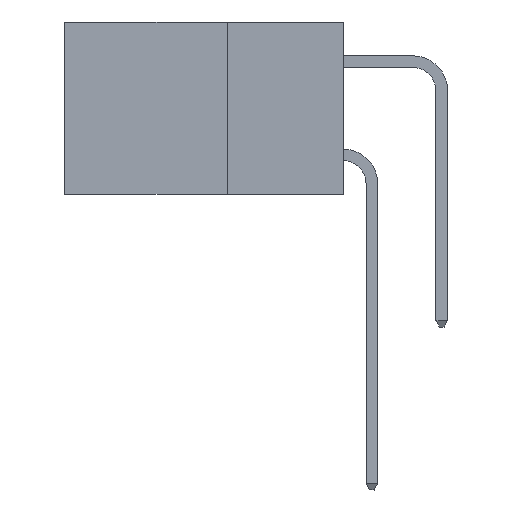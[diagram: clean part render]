
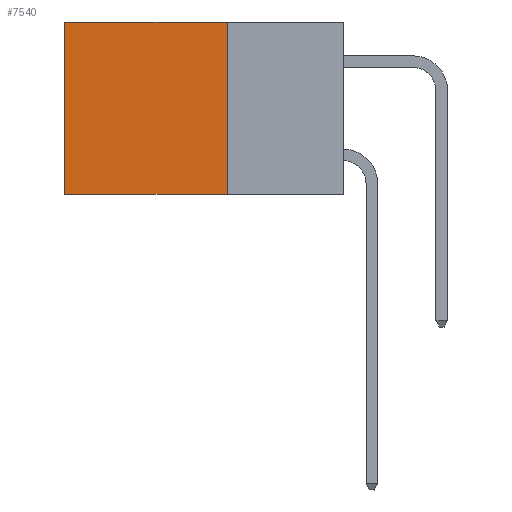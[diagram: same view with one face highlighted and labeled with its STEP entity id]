
A CAD part, left-side view. The second image highlights one B-rep face of the part: STEP entity #7540.
In plain terms, the highlighted planar face has unit normal (-1, 0, 0).
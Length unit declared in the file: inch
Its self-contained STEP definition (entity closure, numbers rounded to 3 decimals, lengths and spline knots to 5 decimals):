
#736 = AXIS2_PLACEMENT_3D ( 'NONE', #2807, #9020, #8856 ) ;
#985 = EDGE_LOOP ( 'NONE', ( #10716, #6815, #7611, #10050 ) ) ;
#1026 = CARTESIAN_POINT ( 'NONE',  ( 0.2615, 0.6, -0.37 ) ) ;
#2457 = VECTOR ( 'NONE', #3982, 39.37008 ) ;
#2609 = CARTESIAN_POINT ( 'NONE',  ( 0.2615, 0.25, 0. ) ) ;
#2657 = CARTESIAN_POINT ( 'NONE',  ( 0.2615, 0.25, -0.37 ) ) ;
#2807 = CARTESIAN_POINT ( 'NONE',  ( 0.2615, 0.25, -0.37 ) ) ;
#3106 = CARTESIAN_POINT ( 'NONE',  ( 0.2615, 0.25, -0.37 ) ) ;
#3982 = DIRECTION ( 'NONE',  ( 0., 0., -1. ) ) ;
#4096 = LINE ( 'NONE', #4791, #9770 ) ;
#4548 = PLANE ( 'NONE',  #736 ) ;
#4791 = CARTESIAN_POINT ( 'NONE',  ( 0.2615, 0.25, 0. ) ) ;
#4793 = VECTOR ( 'NONE', #8929, 39.37008 ) ;
#5202 = CARTESIAN_POINT ( 'NONE',  ( 0.2615, 0.6, 0. ) ) ;
#5238 = VERTEX_POINT ( 'NONE', #2609 ) ;
#5350 = VECTOR ( 'NONE', #6185, 39.37008 ) ;
#5362 = FACE_OUTER_BOUND ( 'NONE', #985, .T. ) ;
#5384 = LINE ( 'NONE', #8878, #4793 ) ;
#5459 = EDGE_CURVE ( 'NONE', #9516, #9732, #5384, .T. ) ;
#6185 = DIRECTION ( 'NONE',  ( 0., 1., 0. ) ) ;
#6481 = VERTEX_POINT ( 'NONE', #9241 ) ;
#6815 = ORIENTED_EDGE ( 'NONE', *, *, #7044, .F. ) ;
#7044 = EDGE_CURVE ( 'NONE', #6481, #9732, #10538, .T. ) ;
#7483 = DIRECTION ( 'NONE',  ( 0., 1., 0. ) ) ;
#7540 = ADVANCED_FACE ( 'NONE', ( #5362 ), #4548, .F. ) ;
#7611 = ORIENTED_EDGE ( 'NONE', *, *, #11112, .F. ) ;
#8856 = DIRECTION ( 'NONE',  ( 0., 0., -1. ) ) ;
#8878 = CARTESIAN_POINT ( 'NONE',  ( 0.2615, 0.6, -0.37 ) ) ;
#8929 = DIRECTION ( 'NONE',  ( 0., 0., -1. ) ) ;
#9020 = DIRECTION ( 'NONE',  ( 1., 0., 0. ) ) ;
#9241 = CARTESIAN_POINT ( 'NONE',  ( 0.2615, 0.25, -0.37 ) ) ;
#9311 = LINE ( 'NONE', #3106, #2457 ) ;
#9516 = VERTEX_POINT ( 'NONE', #5202 ) ;
#9732 = VERTEX_POINT ( 'NONE', #1026 ) ;
#9770 = VECTOR ( 'NONE', #7483, 39.37008 ) ;
#9780 = EDGE_CURVE ( 'NONE', #5238, #9516, #4096, .T. ) ;
#10050 = ORIENTED_EDGE ( 'NONE', *, *, #9780, .T. ) ;
#10538 = LINE ( 'NONE', #2657, #5350 ) ;
#10716 = ORIENTED_EDGE ( 'NONE', *, *, #5459, .T. ) ;
#11112 = EDGE_CURVE ( 'NONE', #5238, #6481, #9311, .T. ) ;
